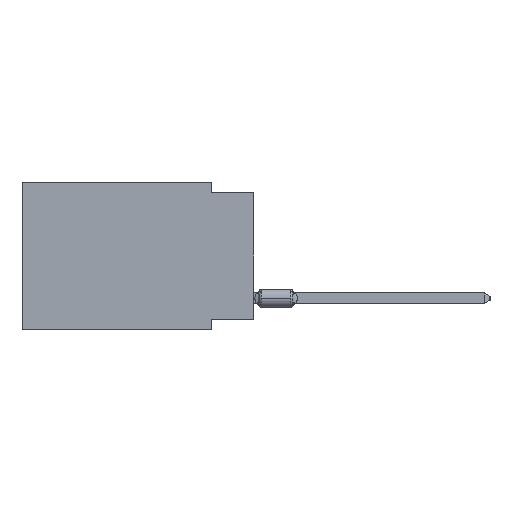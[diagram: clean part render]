
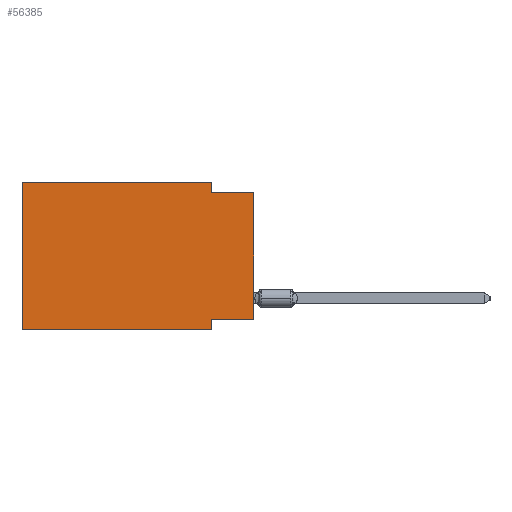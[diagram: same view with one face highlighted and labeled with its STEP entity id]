
A CAD part, left-side view. The second image highlights one B-rep face of the part: STEP entity #56385.
In plain terms, the highlighted planar face has unit normal (-1, 0, 0).
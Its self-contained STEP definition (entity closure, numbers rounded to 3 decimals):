
#293 = CARTESIAN_POINT ( 'NONE',  ( 0., 13.97, 0. ) ) ;
#462 = PLANE ( 'NONE',  #11594 ) ;
#683 = CARTESIAN_POINT ( 'NONE',  ( 0., 0., -8.255 ) ) ;
#743 = CARTESIAN_POINT ( 'NONE',  ( 0., 13.97, 0. ) ) ;
#1700 = EDGE_CURVE ( 'NONE', #9430, #28793, #53295, .T. ) ;
#1807 = VERTEX_POINT ( 'NONE', #71916 ) ;
#3686 = VECTOR ( 'NONE', #70773, 1000. ) ;
#5501 = VERTEX_POINT ( 'NONE', #26393 ) ;
#5583 = DIRECTION ( 'NONE',  ( 0., 0., -1. ) ) ;
#5837 = VECTOR ( 'NONE', #67848, 1000. ) ;
#6964 = VERTEX_POINT ( 'NONE', #11323 ) ;
#8048 = DIRECTION ( 'NONE',  ( 0., -1., 0. ) ) ;
#8687 = LINE ( 'NONE', #65527, #10856 ) ;
#9430 = VERTEX_POINT ( 'NONE', #68844 ) ;
#9749 = EDGE_CURVE ( 'NONE', #5501, #12424, #13512, .T. ) ;
#10263 = LINE ( 'NONE', #743, #65224 ) ;
#10856 = VECTOR ( 'NONE', #22750, 1000. ) ;
#11323 = CARTESIAN_POINT ( 'NONE',  ( 0., 2.54, -8.255 ) ) ;
#11594 = AXIS2_PLACEMENT_3D ( 'NONE', #66912, #44242, #5583 ) ;
#12424 = VERTEX_POINT ( 'NONE', #52758 ) ;
#13512 = LINE ( 'NONE', #58047, #45848 ) ;
#15953 = CARTESIAN_POINT ( 'NONE',  ( 0., 2.54, -8.89 ) ) ;
#16781 = VERTEX_POINT ( 'NONE', #683 ) ;
#18231 = ORIENTED_EDGE ( 'NONE', *, *, #1700, .F. ) ;
#18237 = VECTOR ( 'NONE', #69023, 1000. ) ;
#19145 = ORIENTED_EDGE ( 'NONE', *, *, #23889, .F. ) ;
#22750 = DIRECTION ( 'NONE',  ( 0., 1., 0. ) ) ;
#22980 = DIRECTION ( 'NONE',  ( 0., -1., 0. ) ) ;
#23280 = LINE ( 'NONE', #45563, #5837 ) ;
#23889 = EDGE_CURVE ( 'NONE', #16781, #6964, #8687, .T. ) ;
#23985 = ORIENTED_EDGE ( 'NONE', *, *, #35696, .F. ) ;
#24124 = ORIENTED_EDGE ( 'NONE', *, *, #49393, .F. ) ;
#26393 = CARTESIAN_POINT ( 'NONE',  ( 0., 13.97, -8.89 ) ) ;
#26867 = CARTESIAN_POINT ( 'NONE',  ( 0., 2.54, 0. ) ) ;
#27086 = FACE_OUTER_BOUND ( 'NONE', #61918, .T. ) ;
#27611 = LINE ( 'NONE', #15953, #3686 ) ;
#28793 = VERTEX_POINT ( 'NONE', #62544 ) ;
#29587 = EDGE_CURVE ( 'NONE', #16781, #28793, #23280, .T. ) ;
#29725 = ORIENTED_EDGE ( 'NONE', *, *, #9749, .T. ) ;
#31943 = ORIENTED_EDGE ( 'NONE', *, *, #40813, .F. ) ;
#32998 = ORIENTED_EDGE ( 'NONE', *, *, #64116, .F. ) ;
#33951 = ORIENTED_EDGE ( 'NONE', *, *, #29587, .T. ) ;
#35696 = EDGE_CURVE ( 'NONE', #5501, #1807, #39702, .T. ) ;
#36716 = DIRECTION ( 'NONE',  ( 0., 0., -1. ) ) ;
#36819 = VECTOR ( 'NONE', #45158, 1000. ) ;
#39702 = LINE ( 'NONE', #293, #36819 ) ;
#40813 = EDGE_CURVE ( 'NONE', #1807, #62567, #10263, .T. ) ;
#44242 = DIRECTION ( 'NONE',  ( 1., 0., 0. ) ) ;
#45158 = DIRECTION ( 'NONE',  ( 0., 0., 1. ) ) ;
#45563 = CARTESIAN_POINT ( 'NONE',  ( 0., 0., 0. ) ) ;
#45848 = VECTOR ( 'NONE', #8048, 1000. ) ;
#45938 = VECTOR ( 'NONE', #36716, 1000. ) ;
#49393 = EDGE_CURVE ( 'NONE', #62567, #9430, #69977, .T. ) ;
#52758 = CARTESIAN_POINT ( 'NONE',  ( 0., 2.54, -8.89 ) ) ;
#53295 = LINE ( 'NONE', #58425, #18237 ) ;
#56385 = ADVANCED_FACE ( 'NONE', ( #27086 ), #462, .F. ) ;
#58047 = CARTESIAN_POINT ( 'NONE',  ( 0., 13.97, -8.89 ) ) ;
#58425 = CARTESIAN_POINT ( 'NONE',  ( 0., 0., -0.635 ) ) ;
#61918 = EDGE_LOOP ( 'NONE', ( #33951, #18231, #24124, #31943, #23985, #29725, #32998, #19145 ) ) ;
#62544 = CARTESIAN_POINT ( 'NONE',  ( 0., 0., -0.635 ) ) ;
#62567 = VERTEX_POINT ( 'NONE', #26867 ) ;
#64116 = EDGE_CURVE ( 'NONE', #6964, #12424, #27611, .T. ) ;
#65224 = VECTOR ( 'NONE', #22980, 1000. ) ;
#65527 = CARTESIAN_POINT ( 'NONE',  ( 0., 0., -8.255 ) ) ;
#66912 = CARTESIAN_POINT ( 'NONE',  ( 0., 13.97, 0. ) ) ;
#67848 = DIRECTION ( 'NONE',  ( 0., 0., 1. ) ) ;
#68844 = CARTESIAN_POINT ( 'NONE',  ( 0., 2.54, -0.635 ) ) ;
#69023 = DIRECTION ( 'NONE',  ( 0., -1., 0. ) ) ;
#69977 = LINE ( 'NONE', #70336, #45938 ) ;
#70336 = CARTESIAN_POINT ( 'NONE',  ( 0., 2.54, 0. ) ) ;
#70773 = DIRECTION ( 'NONE',  ( 0., 0., -1. ) ) ;
#71916 = CARTESIAN_POINT ( 'NONE',  ( 0., 13.97, 0. ) ) ;
